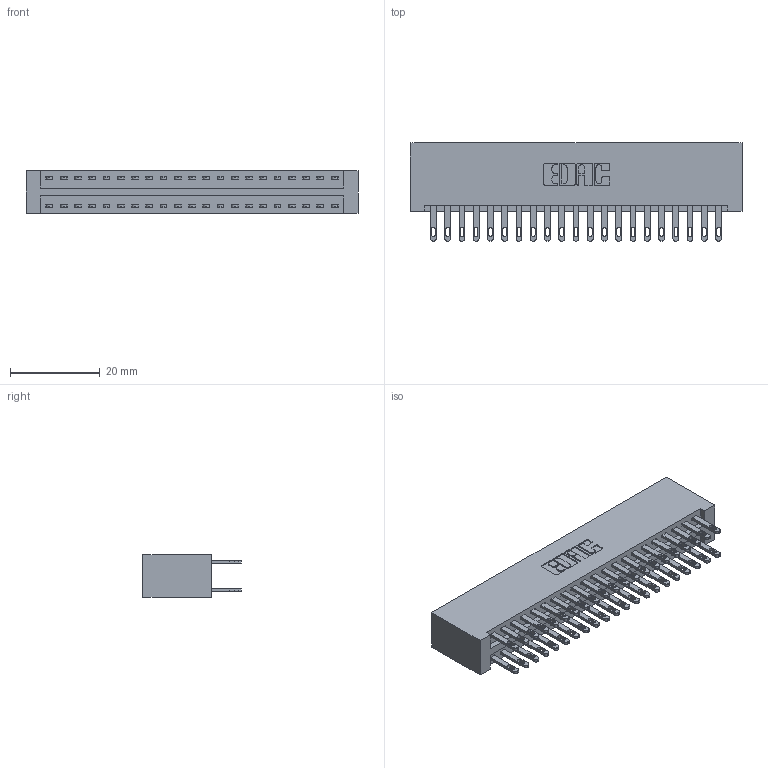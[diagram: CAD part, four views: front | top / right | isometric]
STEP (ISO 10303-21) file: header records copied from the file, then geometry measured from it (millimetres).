
FILE_DESCRIPTION (( 'STEP AP203' ), '1' );
FILE_NAME ('346-042-500-201.STEP', '2018-08-24T12:21:06', ( '' ), ( '' ), 'SwSTEP 2.0', 'SolidWorks 2016', '' );
FILE_SCHEMA (( 'CONFIG_CONTROL_DESIGN' ));
Length unit declared in the file: inch
Products named in the file (3): 346 Part_No Mounting Lugs; 345-292-001_345-293-100; 346-042-500-201
Assembly tree (43 placements, depth 2):
  346-042-500-201
    346 Part_No Mounting Lugs
    345-292-001_345-293-100  x42
Bounding box: 73.91 x 21.84 x 9.4 mm (x, y, z)
Volume: 7746.1 mm3; surface area: 10920.2 mm2
Topology: 43 solids, 43 shells, 2130 faces, 6479 edges, 4318 vertices
Faces by surface type: plane 1290, cylinder 840
Entity records: 16185 total; most frequent: CARTESIAN_POINT 2692, ORIENTED_EDGE 2626, DIRECTION 2421, EDGE_CURVE 1313, VECTOR 1101, LINE 1101, VERTEX_POINT 874, AXIS2_PLACEMENT_3D 660
